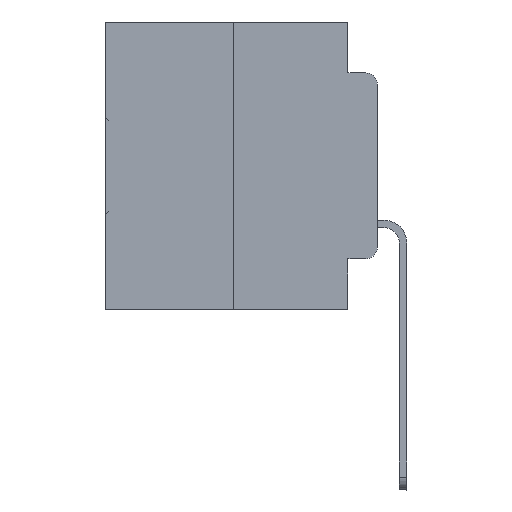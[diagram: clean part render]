
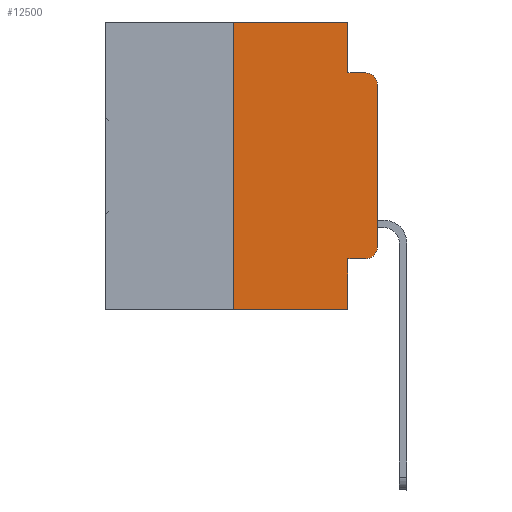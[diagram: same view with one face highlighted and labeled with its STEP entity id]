
A CAD part, left-side view. The second image highlights one B-rep face of the part: STEP entity #12500.
In plain terms, the highlighted planar face has unit normal (-1, 0, 0).
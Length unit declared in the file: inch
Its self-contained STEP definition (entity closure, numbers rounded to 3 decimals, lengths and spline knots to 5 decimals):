
#629 = CARTESIAN_POINT ( 'NONE',  ( 0., 0.02, -0.1085 ) ) ;
#842 = CARTESIAN_POINT ( 'NONE',  ( 0., 0., 0. ) ) ;
#1102 = CIRCLE ( 'NONE', #1644, 0.02 ) ;
#1644 = AXIS2_PLACEMENT_3D ( 'NONE', #629, #10981, #17986 ) ;
#2029 = FACE_OUTER_BOUND ( 'NONE', #20951, .T. ) ;
#2056 = CARTESIAN_POINT ( 'NONE',  ( 0., 0.02, -0.0885 ) ) ;
#2154 = VERTEX_POINT ( 'NONE', #16398 ) ;
#2598 = VERTEX_POINT ( 'NONE', #2056 ) ;
#2802 = LINE ( 'NONE', #20843, #10703 ) ;
#2872 = DIRECTION ( 'NONE',  ( 0., 0., -1. ) ) ;
#3771 = VERTEX_POINT ( 'NONE', #18448 ) ;
#3821 = CARTESIAN_POINT ( 'NONE',  ( 0., 0.051, 0. ) ) ;
#4391 = CARTESIAN_POINT ( 'NONE',  ( 0., 0.051, -0.0885 ) ) ;
#5530 = DIRECTION ( 'NONE',  ( 0., -1., 0. ) ) ;
#5579 = VECTOR ( 'NONE', #21918, 39.37008 ) ;
#5660 = LINE ( 'NONE', #13473, #16387 ) ;
#5888 = VERTEX_POINT ( 'NONE', #23470 ) ;
#6144 = EDGE_CURVE ( 'NONE', #17347, #2598, #22422, .T. ) ;
#6463 = DIRECTION ( 'NONE',  ( 0., 0., -1. ) ) ;
#6961 = LINE ( 'NONE', #17525, #30828 ) ;
#9284 = VERTEX_POINT ( 'NONE', #11018 ) ;
#9932 = CARTESIAN_POINT ( 'NONE',  ( 0., 0.051, -0.0885 ) ) ;
#10156 = DIRECTION ( 'NONE',  ( 0., -1., 0. ) ) ;
#10703 = VECTOR ( 'NONE', #5530, 39.37008 ) ;
#10784 = CARTESIAN_POINT ( 'NONE',  ( 0., 0.25, -0.5 ) ) ;
#10848 = VECTOR ( 'NONE', #10156, 39.37008 ) ;
#10872 = EDGE_CURVE ( 'NONE', #22377, #2598, #1102, .T. ) ;
#10972 = ORIENTED_EDGE ( 'NONE', *, *, #16365, .F. ) ;
#10981 = DIRECTION ( 'NONE',  ( -1., 0., 0. ) ) ;
#11018 = CARTESIAN_POINT ( 'NONE',  ( 0., 0.02, -0.4115 ) ) ;
#11803 = DIRECTION ( 'NONE',  ( 0., 0., -1. ) ) ;
#12500 = ADVANCED_FACE ( 'NONE', ( #2029 ), #21419, .F. ) ;
#13102 = ORIENTED_EDGE ( 'NONE', *, *, #6144, .F. ) ;
#13473 = CARTESIAN_POINT ( 'NONE',  ( 0., 0.051, -0.4115 ) ) ;
#13497 = EDGE_CURVE ( 'NONE', #2154, #17347, #6961, .T. ) ;
#14077 = LINE ( 'NONE', #842, #5579 ) ;
#14961 = ORIENTED_EDGE ( 'NONE', *, *, #13497, .F. ) ;
#15155 = AXIS2_PLACEMENT_3D ( 'NONE', #16551, #32162, #31501 ) ;
#15677 = ORIENTED_EDGE ( 'NONE', *, *, #29266, .T. ) ;
#15720 = ORIENTED_EDGE ( 'NONE', *, *, #25086, .T. ) ;
#16005 = EDGE_CURVE ( 'NONE', #3771, #30981, #22029, .T. ) ;
#16365 = EDGE_CURVE ( 'NONE', #31600, #5888, #27090, .T. ) ;
#16387 = VECTOR ( 'NONE', #23846, 39.37008 ) ;
#16398 = CARTESIAN_POINT ( 'NONE',  ( 0., 0.051, 0. ) ) ;
#16551 = CARTESIAN_POINT ( 'NONE',  ( 0., 0.02, -0.3915 ) ) ;
#16829 = VECTOR ( 'NONE', #32197, 39.37008 ) ;
#17347 = VERTEX_POINT ( 'NONE', #9932 ) ;
#17472 = ORIENTED_EDGE ( 'NONE', *, *, #16005, .F. ) ;
#17525 = CARTESIAN_POINT ( 'NONE',  ( 0., 0.051, 0. ) ) ;
#17986 = DIRECTION ( 'NONE',  ( 0., 0., -1. ) ) ;
#18448 = CARTESIAN_POINT ( 'NONE',  ( 0., 0.051, -0.4115 ) ) ;
#19287 = EDGE_CURVE ( 'NONE', #25258, #22377, #14077, .T. ) ;
#19318 = ORIENTED_EDGE ( 'NONE', *, *, #24515, .T. ) ;
#20167 = ORIENTED_EDGE ( 'NONE', *, *, #19287, .T. ) ;
#20445 = ORIENTED_EDGE ( 'NONE', *, *, #27648, .F. ) ;
#20843 = CARTESIAN_POINT ( 'NONE',  ( 0., 0.473, -0.5 ) ) ;
#20951 = EDGE_LOOP ( 'NONE', ( #20167, #26267, #13102, #14961, #20445, #10972, #19318, #17472, #15677, #15720 ) ) ;
#21254 = CARTESIAN_POINT ( 'NONE',  ( 0., 0.473, 0. ) ) ;
#21419 = PLANE ( 'NONE',  #27725 ) ;
#21918 = DIRECTION ( 'NONE',  ( 0., 0., 1. ) ) ;
#22029 = LINE ( 'NONE', #3821, #31722 ) ;
#22377 = VERTEX_POINT ( 'NONE', #23069 ) ;
#22422 = LINE ( 'NONE', #4391, #10848 ) ;
#23069 = CARTESIAN_POINT ( 'NONE',  ( 0., 0., -0.1085 ) ) ;
#23470 = CARTESIAN_POINT ( 'NONE',  ( 0., 0.25, 0. ) ) ;
#23846 = DIRECTION ( 'NONE',  ( 0., -1., 0. ) ) ;
#24515 = EDGE_CURVE ( 'NONE', #31600, #30981, #2802, .T. ) ;
#24521 = CARTESIAN_POINT ( 'NONE',  ( 0., 0., -0.3915 ) ) ;
#25035 = CARTESIAN_POINT ( 'NONE',  ( 0., 0.25, 0. ) ) ;
#25086 = EDGE_CURVE ( 'NONE', #9284, #25258, #32673, .T. ) ;
#25258 = VERTEX_POINT ( 'NONE', #24521 ) ;
#26267 = ORIENTED_EDGE ( 'NONE', *, *, #10872, .T. ) ;
#27090 = LINE ( 'NONE', #25035, #28490 ) ;
#27648 = EDGE_CURVE ( 'NONE', #5888, #2154, #32027, .T. ) ;
#27725 = AXIS2_PLACEMENT_3D ( 'NONE', #21254, #28717, #2872 ) ;
#28490 = VECTOR ( 'NONE', #30142, 39.37008 ) ;
#28619 = CARTESIAN_POINT ( 'NONE',  ( 0., 0.051, -0.5 ) ) ;
#28717 = DIRECTION ( 'NONE',  ( 1., 0., 0. ) ) ;
#29266 = EDGE_CURVE ( 'NONE', #3771, #9284, #5660, .T. ) ;
#29312 = CARTESIAN_POINT ( 'NONE',  ( 0., 0.473, 0. ) ) ;
#30142 = DIRECTION ( 'NONE',  ( 0., 0., 1. ) ) ;
#30828 = VECTOR ( 'NONE', #6463, 39.37008 ) ;
#30981 = VERTEX_POINT ( 'NONE', #28619 ) ;
#31501 = DIRECTION ( 'NONE',  ( 0., 0., -1. ) ) ;
#31600 = VERTEX_POINT ( 'NONE', #10784 ) ;
#31722 = VECTOR ( 'NONE', #11803, 39.37008 ) ;
#32027 = LINE ( 'NONE', #29312, #16829 ) ;
#32162 = DIRECTION ( 'NONE',  ( -1., 0., 0. ) ) ;
#32197 = DIRECTION ( 'NONE',  ( 0., -1., 0. ) ) ;
#32673 = CIRCLE ( 'NONE', #15155, 0.02 ) ;
